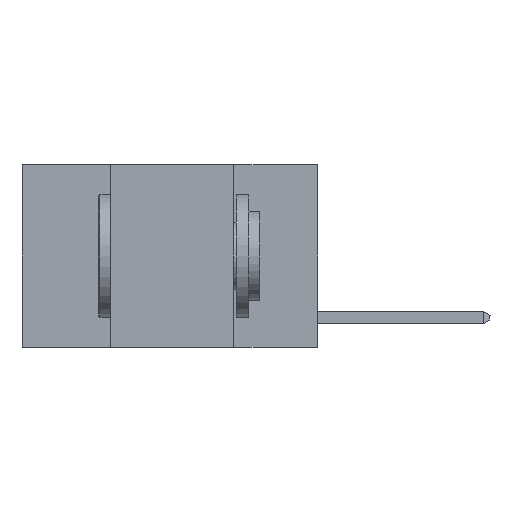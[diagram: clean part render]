
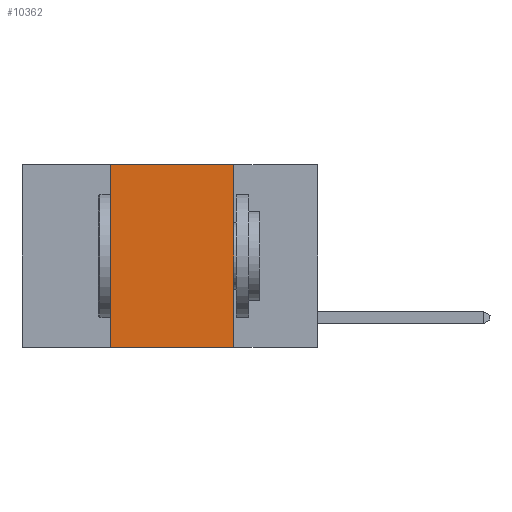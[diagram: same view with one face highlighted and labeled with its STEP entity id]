
A CAD part, left-side view. The second image highlights one B-rep face of the part: STEP entity #10362.
In plain terms, the highlighted planar face has unit normal (-1, 0, 0).
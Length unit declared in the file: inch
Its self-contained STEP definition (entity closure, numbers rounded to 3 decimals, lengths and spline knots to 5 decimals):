
#829 = PLANE ( 'NONE',  #18337 ) ;
#1384 = LINE ( 'NONE', #25414, #11092 ) ;
#1605 = EDGE_CURVE ( 'NONE', #10866, #19314, #18660, .T. ) ;
#1845 = VECTOR ( 'NONE', #20459, 39.37008 ) ;
#2795 = LINE ( 'NONE', #16233, #17954 ) ;
#4560 = ORIENTED_EDGE ( 'NONE', *, *, #1605, .F. ) ;
#4592 = CARTESIAN_POINT ( 'NONE',  ( 0., 0.42, 0. ) ) ;
#4861 = VERTEX_POINT ( 'NONE', #4592 ) ;
#5566 = CARTESIAN_POINT ( 'NONE',  ( 0., 0.17, 0. ) ) ;
#7538 = CARTESIAN_POINT ( 'NONE',  ( 0., 0.17, 0. ) ) ;
#8605 = VERTEX_POINT ( 'NONE', #15603 ) ;
#9546 = CARTESIAN_POINT ( 'NONE',  ( 0., 0.6, 0. ) ) ;
#10362 = ADVANCED_FACE ( 'NONE', ( #13931 ), #829, .F. ) ;
#10866 = VERTEX_POINT ( 'NONE', #5566 ) ;
#11092 = VECTOR ( 'NONE', #23216, 39.37008 ) ;
#11320 = VECTOR ( 'NONE', #27675, 39.37008 ) ;
#11561 = LINE ( 'NONE', #20167, #1845 ) ;
#13675 = ORIENTED_EDGE ( 'NONE', *, *, #25593, .F. ) ;
#13931 = FACE_OUTER_BOUND ( 'NONE', #14030, .T. ) ;
#14030 = EDGE_LOOP ( 'NONE', ( #4560, #13675, #15047, #21372 ) ) ;
#15047 = ORIENTED_EDGE ( 'NONE', *, *, #20023, .F. ) ;
#15603 = CARTESIAN_POINT ( 'NONE',  ( 0., 0.42, -0.37 ) ) ;
#16233 = CARTESIAN_POINT ( 'NONE',  ( 0., 0.42, 0. ) ) ;
#17954 = VECTOR ( 'NONE', #18558, 39.37008 ) ;
#18337 = AXIS2_PLACEMENT_3D ( 'NONE', #9546, #18466, #27035 ) ;
#18466 = DIRECTION ( 'NONE',  ( 1., 0., 0. ) ) ;
#18558 = DIRECTION ( 'NONE',  ( 0., 0., 1. ) ) ;
#18660 = LINE ( 'NONE', #7538, #11320 ) ;
#19314 = VERTEX_POINT ( 'NONE', #21304 ) ;
#20023 = EDGE_CURVE ( 'NONE', #8605, #4861, #2795, .T. ) ;
#20167 = CARTESIAN_POINT ( 'NONE',  ( 0., 0.6, 0. ) ) ;
#20459 = DIRECTION ( 'NONE',  ( 0., -1., 0. ) ) ;
#21304 = CARTESIAN_POINT ( 'NONE',  ( 0., 0.17, -0.37 ) ) ;
#21372 = ORIENTED_EDGE ( 'NONE', *, *, #23174, .T. ) ;
#23174 = EDGE_CURVE ( 'NONE', #8605, #19314, #1384, .T. ) ;
#23216 = DIRECTION ( 'NONE',  ( 0., -1., 0. ) ) ;
#25414 = CARTESIAN_POINT ( 'NONE',  ( 0., 0.6, -0.37 ) ) ;
#25593 = EDGE_CURVE ( 'NONE', #4861, #10866, #11561, .T. ) ;
#27035 = DIRECTION ( 'NONE',  ( 0., 0., -1. ) ) ;
#27675 = DIRECTION ( 'NONE',  ( 0., 0., -1. ) ) ;
